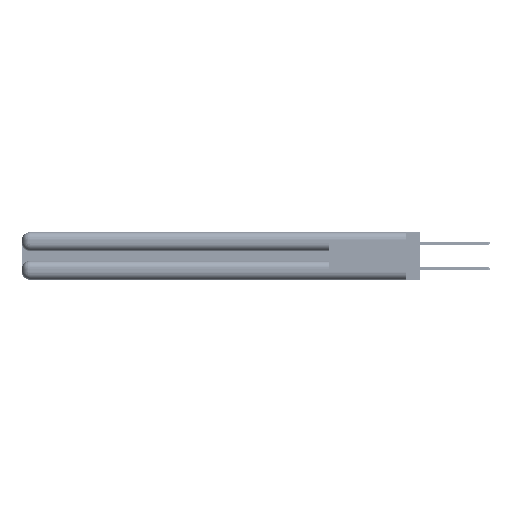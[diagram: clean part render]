
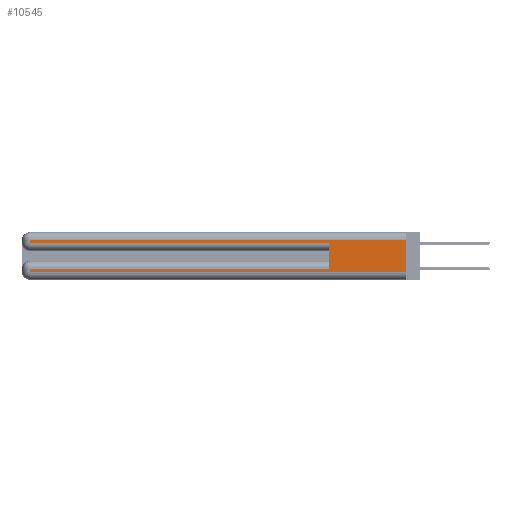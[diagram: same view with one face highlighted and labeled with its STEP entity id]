
A CAD part, left-side view. The second image highlights one B-rep face of the part: STEP entity #10545.
In plain terms, the highlighted planar face has unit normal (-1, 0, 0).
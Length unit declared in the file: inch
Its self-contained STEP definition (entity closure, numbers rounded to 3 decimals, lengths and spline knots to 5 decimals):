
#298 = VERTEX_POINT ( 'NONE', #11131 ) ;
#919 = ORIENTED_EDGE ( 'NONE', *, *, #4102, .T. ) ;
#1083 = LINE ( 'NONE', #35039, #9677 ) ;
#1751 = DIRECTION ( 'NONE',  ( 0., 0., -1. ) ) ;
#3247 = DIRECTION ( 'NONE',  ( 0., 1., 0. ) ) ;
#3642 = CARTESIAN_POINT ( 'NONE',  ( 0., 2.94, 0.37 ) ) ;
#3852 = EDGE_CURVE ( 'NONE', #51119, #298, #33256, .T. ) ;
#4102 = EDGE_CURVE ( 'NONE', #5662, #30594, #25470, .T. ) ;
#4275 = VERTEX_POINT ( 'NONE', #42644 ) ;
#4333 = ORIENTED_EDGE ( 'NONE', *, *, #28859, .T. ) ;
#4690 = LINE ( 'NONE', #3642, #25589 ) ;
#5662 = VERTEX_POINT ( 'NONE', #9091 ) ;
#6236 = ORIENTED_EDGE ( 'NONE', *, *, #46998, .T. ) ;
#6290 = ORIENTED_EDGE ( 'NONE', *, *, #21194, .T. ) ;
#7887 = DIRECTION ( 'NONE',  ( 0., 0., -1. ) ) ;
#9091 = CARTESIAN_POINT ( 'NONE',  ( 0., 0.6, 0.085 ) ) ;
#9677 = VECTOR ( 'NONE', #39209, 39.37008 ) ;
#10235 = CARTESIAN_POINT ( 'NONE',  ( 0., 0., 0.37 ) ) ;
#10545 = ADVANCED_FACE ( 'NONE', ( #41353 ), #41263, .F. ) ;
#11006 = CARTESIAN_POINT ( 'NONE',  ( 0., 0.6, 0.145 ) ) ;
#11131 = CARTESIAN_POINT ( 'NONE',  ( 0., 0., 0.06 ) ) ;
#11425 = ORIENTED_EDGE ( 'NONE', *, *, #3852, .F. ) ;
#12259 = AXIS2_PLACEMENT_3D ( 'NONE', #45387, #20555, #49573 ) ;
#14033 = CARTESIAN_POINT ( 'NONE',  ( 0., 0., 0.31 ) ) ;
#14394 = DIRECTION ( 'NONE',  ( 0., 1., 0. ) ) ;
#15145 = CARTESIAN_POINT ( 'NONE',  ( 0., 2.94, 0.31 ) ) ;
#17779 = EDGE_CURVE ( 'NONE', #4275, #30199, #1083, .T. ) ;
#18506 = VERTEX_POINT ( 'NONE', #52506 ) ;
#20555 = DIRECTION ( 'NONE',  ( 1., 0., 0. ) ) ;
#21194 = EDGE_CURVE ( 'NONE', #30594, #18506, #35425, .T. ) ;
#21516 = VECTOR ( 'NONE', #3247, 39.37008 ) ;
#23319 = LINE ( 'NONE', #14033, #42791 ) ;
#23874 = ORIENTED_EDGE ( 'NONE', *, *, #25839, .T. ) ;
#24998 = DIRECTION ( 'NONE',  ( 0., -1., 0. ) ) ;
#25470 = LINE ( 'NONE', #44741, #21516 ) ;
#25589 = VECTOR ( 'NONE', #7887, 39.37008 ) ;
#25636 = LINE ( 'NONE', #45615, #35348 ) ;
#25839 = EDGE_CURVE ( 'NONE', #42753, #4275, #4690, .T. ) ;
#25992 = CARTESIAN_POINT ( 'NONE',  ( 0., 0., 0.31 ) ) ;
#28859 = EDGE_CURVE ( 'NONE', #18506, #298, #25636, .T. ) ;
#29056 = ORIENTED_EDGE ( 'NONE', *, *, #17779, .T. ) ;
#30199 = VERTEX_POINT ( 'NONE', #37698 ) ;
#30594 = VERTEX_POINT ( 'NONE', #41128 ) ;
#31094 = VECTOR ( 'NONE', #40238, 39.37008 ) ;
#33256 = LINE ( 'NONE', #10235, #42978 ) ;
#34468 = DIRECTION ( 'NONE',  ( 0., 0., -1. ) ) ;
#35039 = CARTESIAN_POINT ( 'NONE',  ( 0., 0., 0.285 ) ) ;
#35348 = VECTOR ( 'NONE', #24998, 39.37008 ) ;
#35425 = LINE ( 'NONE', #42825, #43852 ) ;
#37698 = CARTESIAN_POINT ( 'NONE',  ( 0., 0.6, 0.285 ) ) ;
#39209 = DIRECTION ( 'NONE',  ( 0., -1., 0. ) ) ;
#40238 = DIRECTION ( 'NONE',  ( 0., 0., 1. ) ) ;
#41128 = CARTESIAN_POINT ( 'NONE',  ( 0., 2.94, 0.085 ) ) ;
#41263 = PLANE ( 'NONE',  #12259 ) ;
#41353 = FACE_OUTER_BOUND ( 'NONE', #47122, .T. ) ;
#42644 = CARTESIAN_POINT ( 'NONE',  ( 0., 2.94, 0.285 ) ) ;
#42753 = VERTEX_POINT ( 'NONE', #15145 ) ;
#42791 = VECTOR ( 'NONE', #14394, 39.37008 ) ;
#42825 = CARTESIAN_POINT ( 'NONE',  ( 0., 2.94, 0.37 ) ) ;
#42978 = VECTOR ( 'NONE', #1751, 39.37008 ) ;
#43852 = VECTOR ( 'NONE', #34468, 39.37008 ) ;
#44741 = CARTESIAN_POINT ( 'NONE',  ( 0., 0., 0.085 ) ) ;
#45387 = CARTESIAN_POINT ( 'NONE',  ( 0., 0., 0.37 ) ) ;
#45615 = CARTESIAN_POINT ( 'NONE',  ( 0., 0., 0.06 ) ) ;
#46014 = LINE ( 'NONE', #11006, #31094 ) ;
#46594 = EDGE_CURVE ( 'NONE', #5662, #30199, #46014, .T. ) ;
#46998 = EDGE_CURVE ( 'NONE', #51119, #42753, #23319, .T. ) ;
#47122 = EDGE_LOOP ( 'NONE', ( #11425, #6236, #23874, #29056, #53667, #919, #6290, #4333 ) ) ;
#49573 = DIRECTION ( 'NONE',  ( 0., 0., -1. ) ) ;
#51119 = VERTEX_POINT ( 'NONE', #25992 ) ;
#52506 = CARTESIAN_POINT ( 'NONE',  ( 0., 2.94, 0.06 ) ) ;
#53667 = ORIENTED_EDGE ( 'NONE', *, *, #46594, .F. ) ;
